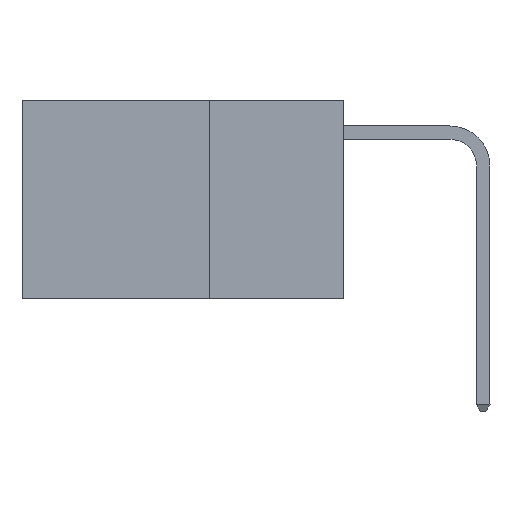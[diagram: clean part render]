
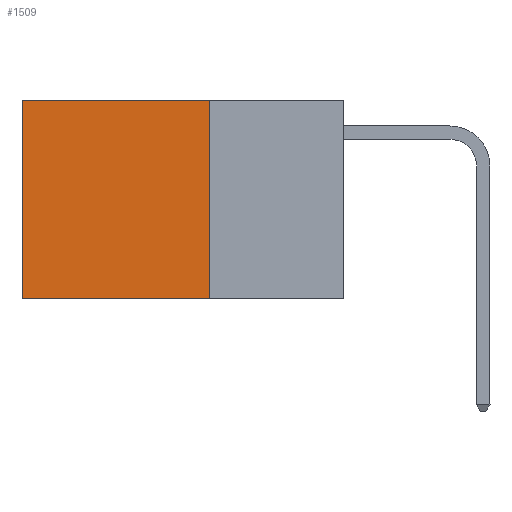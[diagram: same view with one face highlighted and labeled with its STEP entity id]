
A CAD part, left-side view. The second image highlights one B-rep face of the part: STEP entity #1509.
In plain terms, the highlighted planar face has unit normal (-1, 0, 0).
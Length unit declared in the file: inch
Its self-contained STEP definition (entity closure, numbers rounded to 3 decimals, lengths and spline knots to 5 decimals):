
#346 = EDGE_CURVE ( 'NONE', #15238, #12752, #17560, .T. ) ;
#443 = CARTESIAN_POINT ( 'NONE',  ( 0.2625, 0.25, -0.37 ) ) ;
#1509 = ADVANCED_FACE ( 'NONE', ( #7801 ), #24888, .F. ) ;
#2045 = VERTEX_POINT ( 'NONE', #5390 ) ;
#2370 = CARTESIAN_POINT ( 'NONE',  ( 0.2625, 0.25, 0. ) ) ;
#4491 = VECTOR ( 'NONE', #19096, 39.37008 ) ;
#4590 = VERTEX_POINT ( 'NONE', #443 ) ;
#5390 = CARTESIAN_POINT ( 'NONE',  ( 0.2625, 0.6, -0.37 ) ) ;
#5661 = EDGE_CURVE ( 'NONE', #12752, #2045, #19894, .T. ) ;
#6127 = AXIS2_PLACEMENT_3D ( 'NONE', #24581, #24829, #24779 ) ;
#7274 = CARTESIAN_POINT ( 'NONE',  ( 0.2625, 0.25, 0. ) ) ;
#7801 = FACE_OUTER_BOUND ( 'NONE', #11167, .T. ) ;
#8792 = VECTOR ( 'NONE', #21241, 39.37008 ) ;
#9242 = DIRECTION ( 'NONE',  ( 0., 0., -1. ) ) ;
#9556 = ORIENTED_EDGE ( 'NONE', *, *, #19337, .F. ) ;
#11167 = EDGE_LOOP ( 'NONE', ( #19448, #20233, #9556, #22298 ) ) ;
#12455 = VECTOR ( 'NONE', #22860, 39.37008 ) ;
#12752 = VERTEX_POINT ( 'NONE', #18523 ) ;
#15015 = EDGE_CURVE ( 'NONE', #4590, #2045, #24087, .T. ) ;
#15238 = VERTEX_POINT ( 'NONE', #2370 ) ;
#17560 = LINE ( 'NONE', #23716, #12455 ) ;
#18523 = CARTESIAN_POINT ( 'NONE',  ( 0.2625, 0.6, 0. ) ) ;
#19096 = DIRECTION ( 'NONE',  ( 0., 0., -1. ) ) ;
#19337 = EDGE_CURVE ( 'NONE', #15238, #4590, #20795, .T. ) ;
#19372 = CARTESIAN_POINT ( 'NONE',  ( 0.2625, 0.25, -0.37 ) ) ;
#19448 = ORIENTED_EDGE ( 'NONE', *, *, #5661, .T. ) ;
#19894 = LINE ( 'NONE', #20954, #4491 ) ;
#20195 = VECTOR ( 'NONE', #9242, 39.37008 ) ;
#20233 = ORIENTED_EDGE ( 'NONE', *, *, #15015, .F. ) ;
#20795 = LINE ( 'NONE', #7274, #20195 ) ;
#20954 = CARTESIAN_POINT ( 'NONE',  ( 0.2625, 0.6, 0. ) ) ;
#21241 = DIRECTION ( 'NONE',  ( 0., 1., 0. ) ) ;
#22298 = ORIENTED_EDGE ( 'NONE', *, *, #346, .T. ) ;
#22860 = DIRECTION ( 'NONE',  ( 0., 1., 0. ) ) ;
#23716 = CARTESIAN_POINT ( 'NONE',  ( 0.2625, 0.25, 0. ) ) ;
#24087 = LINE ( 'NONE', #19372, #8792 ) ;
#24581 = CARTESIAN_POINT ( 'NONE',  ( 0.2625, 0.25, 0. ) ) ;
#24779 = DIRECTION ( 'NONE',  ( 0., 0., -1. ) ) ;
#24829 = DIRECTION ( 'NONE',  ( 1., 0., 0. ) ) ;
#24888 = PLANE ( 'NONE',  #6127 ) ;
